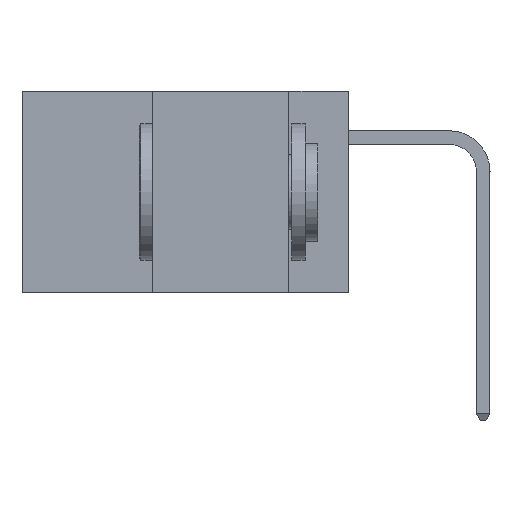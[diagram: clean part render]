
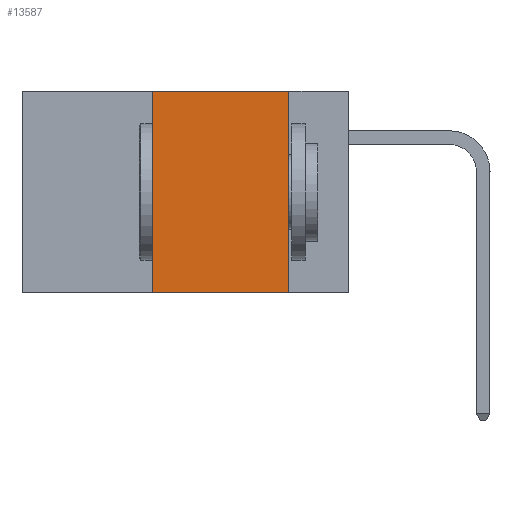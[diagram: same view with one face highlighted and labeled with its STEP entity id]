
A CAD part, left-side view. The second image highlights one B-rep face of the part: STEP entity #13587.
In plain terms, the highlighted planar face has unit normal (-1, 0, 0).
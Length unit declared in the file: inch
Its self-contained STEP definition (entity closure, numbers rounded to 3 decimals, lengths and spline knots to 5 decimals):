
#2102 = ORIENTED_EDGE ( 'NONE', *, *, #22933, .F. ) ;
#2726 = VERTEX_POINT ( 'NONE', #19409 ) ;
#3588 = ORIENTED_EDGE ( 'NONE', *, *, #6478, .F. ) ;
#4517 = EDGE_CURVE ( 'NONE', #16189, #12399, #20582, .T. ) ;
#4854 = VECTOR ( 'NONE', #12423, 39.37008 ) ;
#5029 = ORIENTED_EDGE ( 'NONE', *, *, #4517, .F. ) ;
#5180 = VECTOR ( 'NONE', #14292, 39.37008 ) ;
#5695 = LINE ( 'NONE', #27492, #26916 ) ;
#6478 = EDGE_CURVE ( 'NONE', #2726, #21246, #13256, .T. ) ;
#6733 = PLANE ( 'NONE',  #35115 ) ;
#7535 = EDGE_LOOP ( 'NONE', ( #5029, #2102, #3588, #19180 ) ) ;
#8429 = EDGE_CURVE ( 'NONE', #2726, #12399, #20260, .T. ) ;
#8439 = CARTESIAN_POINT ( 'NONE',  ( 0., 0.11, 0. ) ) ;
#9673 = DIRECTION ( 'NONE',  ( 0., 0., -1. ) ) ;
#12106 = CARTESIAN_POINT ( 'NONE',  ( 0., 0.36, 0. ) ) ;
#12399 = VERTEX_POINT ( 'NONE', #17813 ) ;
#12423 = DIRECTION ( 'NONE',  ( 0., -1., 0. ) ) ;
#13256 = LINE ( 'NONE', #14163, #28504 ) ;
#13587 = ADVANCED_FACE ( 'NONE', ( #25302 ), #6733, .F. ) ;
#14163 = CARTESIAN_POINT ( 'NONE',  ( 0., 0.36, 0. ) ) ;
#14292 = DIRECTION ( 'NONE',  ( 0., 0., -1. ) ) ;
#16189 = VERTEX_POINT ( 'NONE', #30848 ) ;
#17813 = CARTESIAN_POINT ( 'NONE',  ( 0., 0.11, -0.37 ) ) ;
#18171 = CARTESIAN_POINT ( 'NONE',  ( 0., 0.6, -0.37 ) ) ;
#19180 = ORIENTED_EDGE ( 'NONE', *, *, #8429, .T. ) ;
#19409 = CARTESIAN_POINT ( 'NONE',  ( 0., 0.36, -0.37 ) ) ;
#20260 = LINE ( 'NONE', #18171, #4854 ) ;
#20582 = LINE ( 'NONE', #8439, #5180 ) ;
#21154 = CARTESIAN_POINT ( 'NONE',  ( 0., 0.6, 0. ) ) ;
#21246 = VERTEX_POINT ( 'NONE', #12106 ) ;
#22933 = EDGE_CURVE ( 'NONE', #21246, #16189, #5695, .T. ) ;
#25302 = FACE_OUTER_BOUND ( 'NONE', #7535, .T. ) ;
#26898 = DIRECTION ( 'NONE',  ( 1., 0., 0. ) ) ;
#26916 = VECTOR ( 'NONE', #36042, 39.37008 ) ;
#27492 = CARTESIAN_POINT ( 'NONE',  ( 0., 0.6, 0. ) ) ;
#28504 = VECTOR ( 'NONE', #34127, 39.37008 ) ;
#30848 = CARTESIAN_POINT ( 'NONE',  ( 0., 0.11, 0. ) ) ;
#34127 = DIRECTION ( 'NONE',  ( 0., 0., 1. ) ) ;
#35115 = AXIS2_PLACEMENT_3D ( 'NONE', #21154, #26898, #9673 ) ;
#36042 = DIRECTION ( 'NONE',  ( 0., -1., 0. ) ) ;
